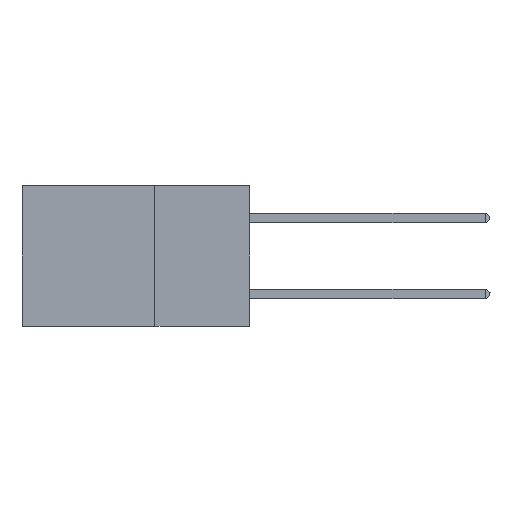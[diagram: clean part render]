
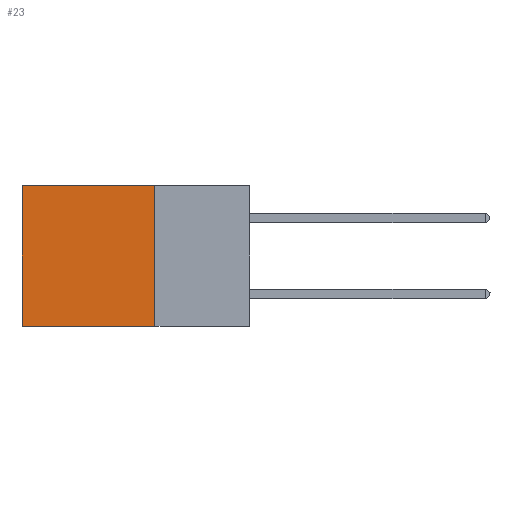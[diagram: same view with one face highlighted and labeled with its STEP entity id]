
A CAD part, left-side view. The second image highlights one B-rep face of the part: STEP entity #23.
In plain terms, the highlighted planar face has unit normal (-1, 0, 0).
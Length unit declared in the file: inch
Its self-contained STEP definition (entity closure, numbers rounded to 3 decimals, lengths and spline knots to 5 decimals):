
#23 = ADVANCED_FACE ( 'NONE', ( #15955 ), #14224, .F. ) ;
#1251 = CARTESIAN_POINT ( 'NONE',  ( 0.2875, 0.25, 0. ) ) ;
#2021 = ORIENTED_EDGE ( 'NONE', *, *, #2836, .F. ) ;
#2836 = EDGE_CURVE ( 'NONE', #21298, #9886, #7345, .T. ) ;
#3372 = LINE ( 'NONE', #1251, #3536 ) ;
#3536 = VECTOR ( 'NONE', #15335, 39.37008 ) ;
#4866 = EDGE_CURVE ( 'NONE', #13696, #17278, #8985, .T. ) ;
#5892 = VECTOR ( 'NONE', #12219, 39.37008 ) ;
#6111 = CARTESIAN_POINT ( 'NONE',  ( 0.2875, 0.25, -0.37 ) ) ;
#6324 = ORIENTED_EDGE ( 'NONE', *, *, #14991, .T. ) ;
#6758 = EDGE_LOOP ( 'NONE', ( #6324, #2021, #18560, #8446 ) ) ;
#7345 = LINE ( 'NONE', #6111, #5892 ) ;
#7533 = CARTESIAN_POINT ( 'NONE',  ( 0.2875, 0.25, 0. ) ) ;
#8446 = ORIENTED_EDGE ( 'NONE', *, *, #4866, .T. ) ;
#8491 = CARTESIAN_POINT ( 'NONE',  ( 0.2875, 0.6, 0. ) ) ;
#8985 = LINE ( 'NONE', #9242, #10989 ) ;
#9242 = CARTESIAN_POINT ( 'NONE',  ( 0.2875, 0.25, 0. ) ) ;
#9719 = EDGE_CURVE ( 'NONE', #13696, #21298, #3372, .T. ) ;
#9821 = DIRECTION ( 'NONE',  ( 1., 0., 0. ) ) ;
#9886 = VERTEX_POINT ( 'NONE', #10253 ) ;
#10253 = CARTESIAN_POINT ( 'NONE',  ( 0.2875, 0.6, -0.37 ) ) ;
#10989 = VECTOR ( 'NONE', #17370, 39.37008 ) ;
#12219 = DIRECTION ( 'NONE',  ( 0., 1., 0. ) ) ;
#13406 = AXIS2_PLACEMENT_3D ( 'NONE', #18089, #9821, #23804 ) ;
#13696 = VERTEX_POINT ( 'NONE', #7533 ) ;
#13797 = DIRECTION ( 'NONE',  ( 0., 0., -1. ) ) ;
#13918 = LINE ( 'NONE', #23770, #19377 ) ;
#14224 = PLANE ( 'NONE',  #13406 ) ;
#14991 = EDGE_CURVE ( 'NONE', #17278, #9886, #13918, .T. ) ;
#15335 = DIRECTION ( 'NONE',  ( 0., 0., -1. ) ) ;
#15955 = FACE_OUTER_BOUND ( 'NONE', #6758, .T. ) ;
#17278 = VERTEX_POINT ( 'NONE', #8491 ) ;
#17370 = DIRECTION ( 'NONE',  ( 0., 1., 0. ) ) ;
#18089 = CARTESIAN_POINT ( 'NONE',  ( 0.2875, 0.25, 0. ) ) ;
#18560 = ORIENTED_EDGE ( 'NONE', *, *, #9719, .F. ) ;
#19377 = VECTOR ( 'NONE', #13797, 39.37008 ) ;
#21071 = CARTESIAN_POINT ( 'NONE',  ( 0.2875, 0.25, -0.37 ) ) ;
#21298 = VERTEX_POINT ( 'NONE', #21071 ) ;
#23770 = CARTESIAN_POINT ( 'NONE',  ( 0.2875, 0.6, 0. ) ) ;
#23804 = DIRECTION ( 'NONE',  ( 0., 0., -1. ) ) ;
